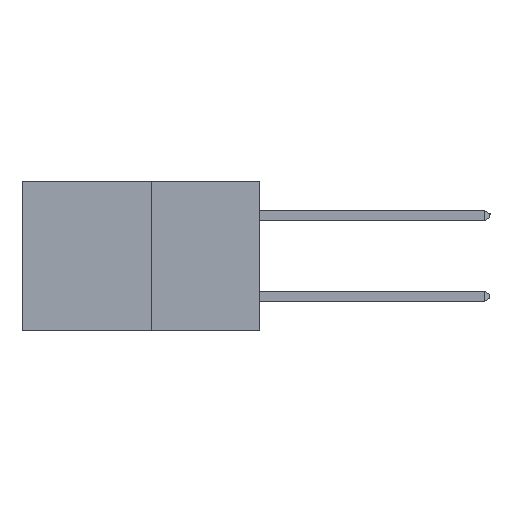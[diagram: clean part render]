
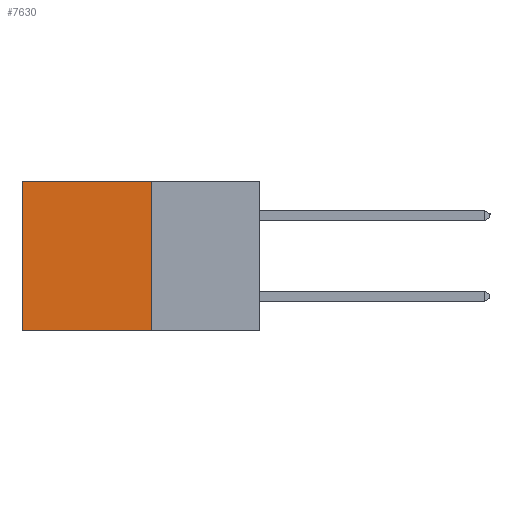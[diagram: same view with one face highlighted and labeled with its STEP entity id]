
A CAD part, left-side view. The second image highlights one B-rep face of the part: STEP entity #7630.
In plain terms, the highlighted planar face has unit normal (-1, 0, 0).
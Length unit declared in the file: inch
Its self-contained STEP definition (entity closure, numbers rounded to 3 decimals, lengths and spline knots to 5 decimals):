
#353 = AXIS2_PLACEMENT_3D ( 'NONE', #1080, #8412, #2128 ) ;
#685 = LINE ( 'NONE', #12291, #5939 ) ;
#1028 = VERTEX_POINT ( 'NONE', #10470 ) ;
#1080 = CARTESIAN_POINT ( 'NONE',  ( 0.277, 0.27, -0.37 ) ) ;
#1304 = VECTOR ( 'NONE', #5222, 39.37008 ) ;
#1694 = VERTEX_POINT ( 'NONE', #11513 ) ;
#1823 = DIRECTION ( 'NONE',  ( 0., 1., 0. ) ) ;
#2128 = DIRECTION ( 'NONE',  ( 0., 0., -1. ) ) ;
#2557 = CARTESIAN_POINT ( 'NONE',  ( 0.277, 0.27, 0. ) ) ;
#2883 = EDGE_LOOP ( 'NONE', ( #10059, #11028, #12036, #5321 ) ) ;
#3099 = VERTEX_POINT ( 'NONE', #12451 ) ;
#3611 = DIRECTION ( 'NONE',  ( 0., 1., 0. ) ) ;
#3873 = VERTEX_POINT ( 'NONE', #9371 ) ;
#4374 = EDGE_CURVE ( 'NONE', #3099, #1028, #685, .T. ) ;
#5216 = LINE ( 'NONE', #2557, #10453 ) ;
#5222 = DIRECTION ( 'NONE',  ( 0., 0., -1. ) ) ;
#5321 = ORIENTED_EDGE ( 'NONE', *, *, #7257, .T. ) ;
#5762 = EDGE_CURVE ( 'NONE', #3873, #3099, #12473, .T. ) ;
#5854 = FACE_OUTER_BOUND ( 'NONE', #2883, .T. ) ;
#5939 = VECTOR ( 'NONE', #1823, 39.37008 ) ;
#7257 = EDGE_CURVE ( 'NONE', #3873, #1694, #5216, .T. ) ;
#7355 = PLANE ( 'NONE',  #353 ) ;
#7485 = DIRECTION ( 'NONE',  ( 0., 0., -1. ) ) ;
#7630 = ADVANCED_FACE ( 'NONE', ( #5854 ), #7355, .F. ) ;
#8412 = DIRECTION ( 'NONE',  ( 1., 0., 0. ) ) ;
#9068 = VECTOR ( 'NONE', #7485, 39.37008 ) ;
#9371 = CARTESIAN_POINT ( 'NONE',  ( 0.277, 0.27, 0. ) ) ;
#10059 = ORIENTED_EDGE ( 'NONE', *, *, #10115, .T. ) ;
#10115 = EDGE_CURVE ( 'NONE', #1694, #1028, #11856, .T. ) ;
#10453 = VECTOR ( 'NONE', #3611, 39.37008 ) ;
#10470 = CARTESIAN_POINT ( 'NONE',  ( 0.277, 0.59, -0.37 ) ) ;
#11028 = ORIENTED_EDGE ( 'NONE', *, *, #4374, .F. ) ;
#11513 = CARTESIAN_POINT ( 'NONE',  ( 0.277, 0.59, 0. ) ) ;
#11856 = LINE ( 'NONE', #12738, #9068 ) ;
#12036 = ORIENTED_EDGE ( 'NONE', *, *, #5762, .F. ) ;
#12291 = CARTESIAN_POINT ( 'NONE',  ( 0.277, 0.27, -0.37 ) ) ;
#12451 = CARTESIAN_POINT ( 'NONE',  ( 0.277, 0.27, -0.37 ) ) ;
#12473 = LINE ( 'NONE', #12558, #1304 ) ;
#12558 = CARTESIAN_POINT ( 'NONE',  ( 0.277, 0.27, -0.37 ) ) ;
#12738 = CARTESIAN_POINT ( 'NONE',  ( 0.277, 0.59, -0.37 ) ) ;
